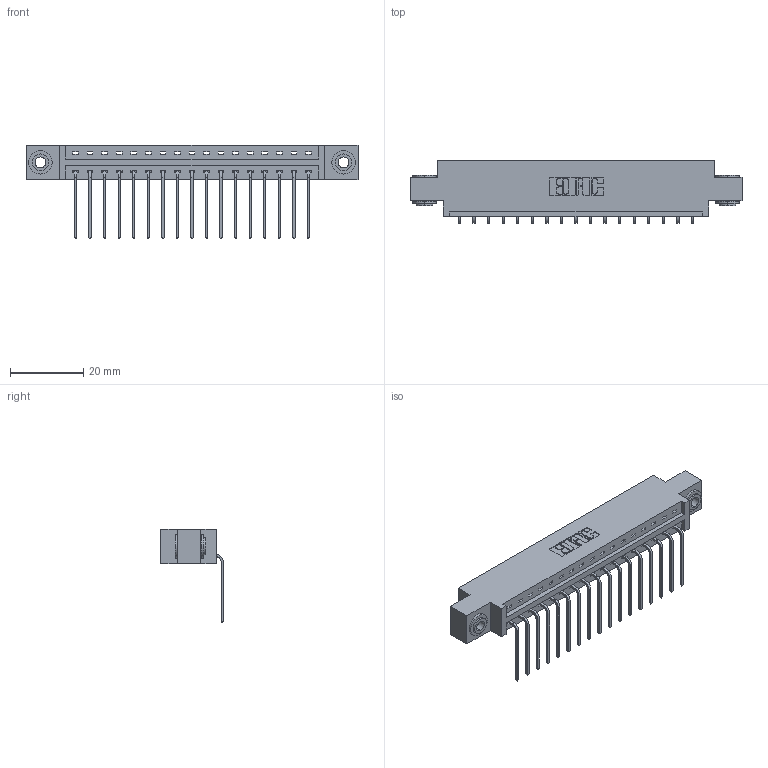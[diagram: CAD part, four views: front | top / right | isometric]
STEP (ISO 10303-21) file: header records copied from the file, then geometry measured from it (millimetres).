
FILE_DESCRIPTION (( 'STEP AP203' ), '1' );
FILE_NAME ('337-017-559-603.STEP', '2018-08-04T22:47:43', ( '' ), ( '' ), 'SwSTEP 2.0', 'SolidWorks 2016', '' );
FILE_SCHEMA (( 'CONFIG_CONTROL_DESIGN' ));
Length unit declared in the file: inch
Products named in the file (4): 337 Part_0.170 Offset - 0.156 Dia-TH; 345-292-001_558 559 Tail - 1; 345-250-002_345-250-002-102; 337-017-559-603
Assembly tree (20 placements, depth 2):
  337-017-559-603
    337 Part_0.170 Offset - 0.156 Dia-TH
    345-292-001_558 559 Tail - 1  x17
    345-250-002_345-250-002-102  x2
Bounding box: 90.37 x 17.09 x 25.53 mm (x, y, z)
Volume: 9038.5 mm3; surface area: 9878.3 mm2
Topology: 20 solids, 20 shells, 1244 faces, 3697 edges, 2438 vertices
Faces by surface type: plane 900, cylinder 336, cone 8
Entity records: 16736 total; most frequent: CARTESIAN_POINT 2892, ORIENTED_EDGE 2838, DIRECTION 2519, EDGE_CURVE 1419, LINE 1267, VECTOR 1267, VERTEX_POINT 942, AXIS2_PLACEMENT_3D 626
